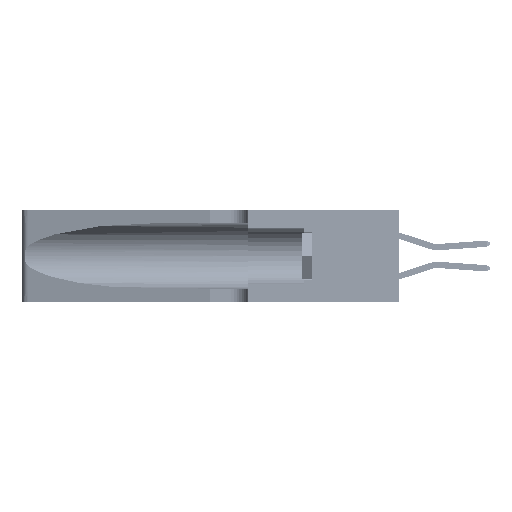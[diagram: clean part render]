
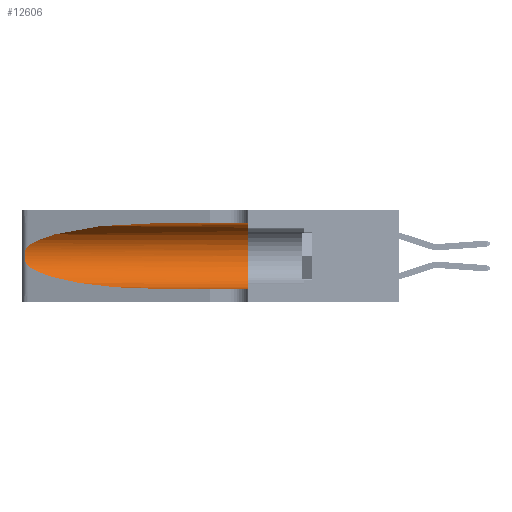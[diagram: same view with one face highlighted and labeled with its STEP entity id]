
A CAD part, left-side view. The second image highlights one B-rep face of the part: STEP entity #12606.
In plain terms, the highlighted cylindrical face has radius 3.308 mm (diameter 6.617 mm), a partial arc.
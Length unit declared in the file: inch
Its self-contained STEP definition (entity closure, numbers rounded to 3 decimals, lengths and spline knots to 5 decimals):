
#38 = LINE ( 'NONE', #27038, #31879 ) ;
#1288 = CARTESIAN_POINT ( 'NONE',  ( 0.25487, 1.22718, 0.22369 ) ) ;
#1476 = CARTESIAN_POINT ( 'NONE',  ( 0.1305, 1.61858, 0.185 ) ) ;
#1855 = CARTESIAN_POINT ( 'NONE',  ( 0.25555, 1.22993, 0.14849 ) ) ;
#2179 = CARTESIAN_POINT ( 'NONE',  ( 0.25487, 1.22718, 0.22369 ) ) ;
#4765 = CIRCLE ( 'NONE', #34311, 0.13025 ) ;
#5314 = EDGE_CURVE ( 'NONE', #10865, #36948, #38, .T. ) ;
#6067 = CARTESIAN_POINT ( 'NONE',  ( 0.1305, 0.72297, 0.31525 ) ) ;
#6739 = LINE ( 'NONE', #16184, #25789 ) ;
#8073 = CARTESIAN_POINT ( 'NONE',  ( 0.2373, 1.15595, 0.08982 ) ) ;
#8420 = VERTEX_POINT ( 'NONE', #38206 ) ;
#10016 = CARTESIAN_POINT ( 'NONE',  ( 0.1305, 0.72297, 0.31525 ) ) ;
#10865 = VERTEX_POINT ( 'NONE', #10016 ) ;
#11206 = CARTESIAN_POINT ( 'NONE',  ( 0.1305, 0.72297, 0.05475 ) ) ;
#11696 = DIRECTION ( 'NONE',  ( 0., 1., 0. ) ) ;
#12472 = CARTESIAN_POINT ( 'NONE',  ( 0.25555, 1.22994, 0.2215 ) ) ;
#12606 = ADVANCED_FACE ( 'NONE', ( #32944 ), #29554, .F. ) ;
#12621 = CARTESIAN_POINT ( 'NONE',  ( 0.25789, 1.23486, 0.15765 ) ) ;
#13067 = CARTESIAN_POINT ( 'NONE',  ( 0.25487, 1.22718, 0.22369 ) ) ;
#13205 = ORIENTED_EDGE ( 'NONE', *, *, #5314, .F. ) ;
#13644 = EDGE_CURVE ( 'NONE', #26947, #30091, #36353, .T. ) ;
#14998 = EDGE_CURVE ( 'NONE', #36948, #8420, #4765, .T. ) ;
#15751 = EDGE_CURVE ( 'NONE', #30091, #8420, #6739, .T. ) ;
#16184 = CARTESIAN_POINT ( 'NONE',  ( 0.1305, 1.61858, 0.05475 ) ) ;
#18551 = CARTESIAN_POINT ( 'NONE',  ( 0.18966, 0.96281, 0.05475 ) ) ;
#19667 = CARTESIAN_POINT ( 'NONE',  ( 0.25639, 1.23186, 0.15144 ) ) ;
#19811 = CARTESIAN_POINT ( 'NONE',  ( 0.25787, 1.23484, 0.2124 ) ) ;
#22837 = CARTESIAN_POINT ( 'NONE',  ( 0.1305, 0.35, 0.185 ) ) ;
#23599 = CARTESIAN_POINT ( 'NONE',  ( 0.26018, 1.23835, 0.19895 ) ) ;
#23915 = CARTESIAN_POINT ( 'NONE',  ( 0.2373, 1.15595, 0.28018 ) ) ;
#24018 = EDGE_CURVE ( 'NONE', #10865, #30097, #32892, .T. ) ;
#24718 = ORIENTED_EDGE ( 'NONE', *, *, #32779, .T. ) ;
#25603 = CARTESIAN_POINT ( 'NONE',  ( 0.25487, 1.22718, 0.14631 ) ) ;
#25789 = VECTOR ( 'NONE', #38060, 39.37008 ) ;
#26059 = CARTESIAN_POINT ( 'NONE',  ( 0.1305, 0.35, 0.31525 ) ) ;
#26859 = CARTESIAN_POINT ( 'NONE',  ( 0.26017, 1.23833, 0.17102 ) ) ;
#26947 = VERTEX_POINT ( 'NONE', #46080 ) ;
#27038 = CARTESIAN_POINT ( 'NONE',  ( 0.1305, 1.61858, 0.31525 ) ) ;
#27166 = B_SPLINE_CURVE_WITH_KNOTS ( 'NONE', 3,
 ( #13067, #12472, #27301, #19811, #38095, #23599, #37508, #41241, #26859, #41092, #12621, #19667, #1855, #37947 ),
 .UNSPECIFIED., .F., .F.,
 ( 4, 2, 2, 2, 2, 2, 4 ),
 ( 0., 0.00027, 0.00053, 0.00107, 0.0016, 0.00187, 0.00214 ),
 .UNSPECIFIED. ) ;
#27301 = CARTESIAN_POINT ( 'NONE',  ( 0.25639, 1.23184, 0.21858 ) ) ;
#29554 = CYLINDRICAL_SURFACE ( 'NONE', #35133, 0.13025 ) ;
#30091 = VERTEX_POINT ( 'NONE', #40692 ) ;
#30097 = VERTEX_POINT ( 'NONE', #1288 ) ;
#31879 = VECTOR ( 'NONE', #43942, 39.37008 ) ;
#32779 = EDGE_CURVE ( 'NONE', #30097, #26947, #27166, .T. ) ;
#32892 =( BOUNDED_CURVE ( )  B_SPLINE_CURVE ( 3, ( #6067, #45021, #23915, #2179 ),
 .UNSPECIFIED., .F., .F. ) 
 B_SPLINE_CURVE_WITH_KNOTS ( ( 4, 4 ),
 ( 1.5708, 2.84003 ),
 .UNSPECIFIED. ) 
 CURVE ( )  GEOMETRIC_REPRESENTATION_ITEM ( )  RATIONAL_B_SPLINE_CURVE ( ( 1., 0.87, 0.87, 1. ) ) 
 REPRESENTATION_ITEM ( '' )  );
#32944 = FACE_OUTER_BOUND ( 'NONE', #45214, .T. ) ;
#34311 = AXIS2_PLACEMENT_3D ( 'NONE', #22837, #11696, #44089 ) ;
#35133 = AXIS2_PLACEMENT_3D ( 'NONE', #1476, #37734, #40875 ) ;
#36353 =( BOUNDED_CURVE ( )  B_SPLINE_CURVE ( 3, ( #25603, #8073, #18551, #11206 ),
 .UNSPECIFIED., .F., .F. ) 
 B_SPLINE_CURVE_WITH_KNOTS ( ( 4, 4 ),
 ( 3.44316, 4.71239 ),
 .UNSPECIFIED. ) 
 CURVE ( )  GEOMETRIC_REPRESENTATION_ITEM ( )  RATIONAL_B_SPLINE_CURVE ( ( 1., 0.87, 0.87, 1. ) ) 
 REPRESENTATION_ITEM ( '' )  );
#36948 = VERTEX_POINT ( 'NONE', #26059 ) ;
#36998 = ORIENTED_EDGE ( 'NONE', *, *, #14998, .F. ) ;
#37508 = CARTESIAN_POINT ( 'NONE',  ( 0.26075, 1.23896, 0.19203 ) ) ;
#37734 = DIRECTION ( 'NONE',  ( 0., -1., 0. ) ) ;
#37947 = CARTESIAN_POINT ( 'NONE',  ( 0.25487, 1.22718, 0.14631 ) ) ;
#38060 = DIRECTION ( 'NONE',  ( 0., -1., 0. ) ) ;
#38095 = CARTESIAN_POINT ( 'NONE',  ( 0.25854, 1.2359, 0.20912 ) ) ;
#38206 = CARTESIAN_POINT ( 'NONE',  ( 0.1305, 0.35, 0.05475 ) ) ;
#39969 = ORIENTED_EDGE ( 'NONE', *, *, #24018, .T. ) ;
#40692 = CARTESIAN_POINT ( 'NONE',  ( 0.1305, 0.72297, 0.05475 ) ) ;
#40875 = DIRECTION ( 'NONE',  ( 0., 0., -1. ) ) ;
#41092 = CARTESIAN_POINT ( 'NONE',  ( 0.25856, 1.23593, 0.16098 ) ) ;
#41241 = CARTESIAN_POINT ( 'NONE',  ( 0.26075, 1.23896, 0.178 ) ) ;
#41643 = ORIENTED_EDGE ( 'NONE', *, *, #15751, .T. ) ;
#43942 = DIRECTION ( 'NONE',  ( 0., -1., 0. ) ) ;
#44089 = DIRECTION ( 'NONE',  ( 0., 0., 1. ) ) ;
#44346 = ORIENTED_EDGE ( 'NONE', *, *, #13644, .T. ) ;
#45021 = CARTESIAN_POINT ( 'NONE',  ( 0.18966, 0.96281, 0.31525 ) ) ;
#45214 = EDGE_LOOP ( 'NONE', ( #39969, #24718, #44346, #41643, #36998, #13205 ) ) ;
#46080 = CARTESIAN_POINT ( 'NONE',  ( 0.25487, 1.22718, 0.14631 ) ) ;
